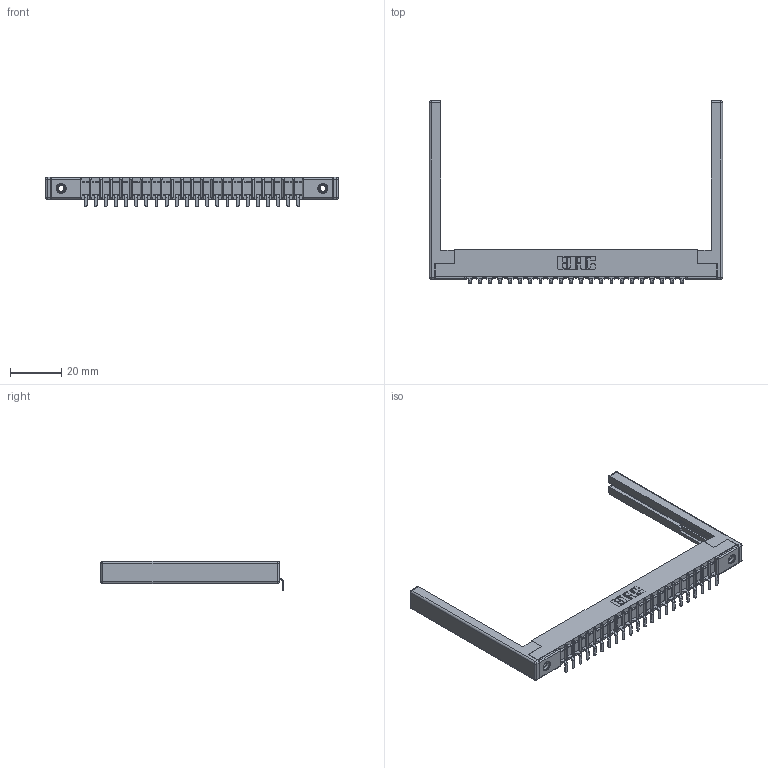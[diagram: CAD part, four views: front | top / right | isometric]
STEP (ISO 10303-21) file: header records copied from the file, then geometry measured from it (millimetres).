
FILE_DESCRIPTION (( 'STEP AP203' ), '1' );
FILE_NAME ('307-022-553-168.STEP', '2019-09-05T00:09:01', ( '' ), ( '' ), 'SwSTEP 2.0', 'SolidWorks 2016', '' );
FILE_SCHEMA (( 'CONFIG_CONTROL_DESIGN' ));
Length unit declared in the file: inch
Products named in the file (5): 307-220-068; 307-022-553-168; 345-250-001_345-250-001-102; 307 Part_.156 Dia Mounting Holes; 307-290-002_553
Assembly tree (27 placements, depth 2):
  307-022-553-168
    307 Part_.156 Dia Mounting Holes
    307-290-002_553  x22
    307-220-068  x2
    345-250-001_345-250-001-102  x2
Bounding box: 114.6 x 71.29 x 11.51 mm (x, y, z)
Volume: 12124.7 mm3; surface area: 17788.3 mm2
Topology: 27 solids, 27 shells, 2011 faces, 6081 edges, 3970 vertices
Faces by surface type: plane 1192, cylinder 749, sphere 54, cone 12, torus 4
Entity records: 24939 total; most frequent: CARTESIAN_POINT 4169, ORIENTED_EDGE 4148, DIRECTION 4078, EDGE_CURVE 2074, LINE 1576, VECTOR 1576, VERTEX_POINT 1342, AXIS2_PLACEMENT_3D 1251
